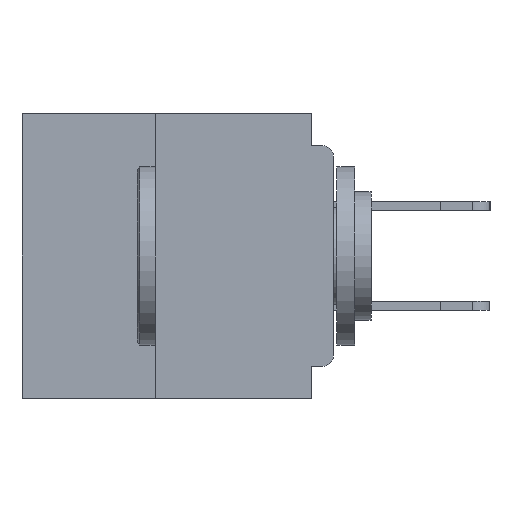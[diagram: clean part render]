
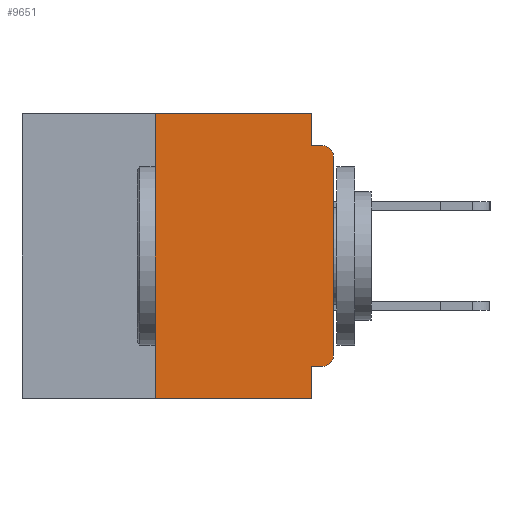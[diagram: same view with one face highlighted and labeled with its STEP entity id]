
A CAD part, left-side view. The second image highlights one B-rep face of the part: STEP entity #9651.
In plain terms, the highlighted planar face has unit normal (-1, 0, 0).
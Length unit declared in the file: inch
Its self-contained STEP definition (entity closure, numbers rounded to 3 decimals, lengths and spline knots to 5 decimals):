
#902 = VECTOR ( 'NONE', #10446, 39.37008 ) ;
#957 = EDGE_CURVE ( 'NONE', #3552, #12985, #12526, .T. ) ;
#1160 = DIRECTION ( 'NONE',  ( 0., 0., -1. ) ) ;
#1739 = EDGE_CURVE ( 'NONE', #25780, #27255, #29302, .T. ) ;
#3304 = CARTESIAN_POINT ( 'NONE',  ( 0., 0.437, 0. ) ) ;
#3520 = CIRCLE ( 'NONE', #38357, 0.015 ) ;
#3552 = VERTEX_POINT ( 'NONE', #10117 ) ;
#4319 = ORIENTED_EDGE ( 'NONE', *, *, #46952, .T. ) ;
#4646 = CIRCLE ( 'NONE', #32870, 0.015 ) ;
#4761 = CARTESIAN_POINT ( 'NONE',  ( 0., 0.437, 0. ) ) ;
#5683 = DIRECTION ( 'NONE',  ( 0., 0., 1. ) ) ;
#7208 = VECTOR ( 'NONE', #29849, 39.37008 ) ;
#7332 = DIRECTION ( 'NONE',  ( 0., 0., -1. ) ) ;
#8312 = ORIENTED_EDGE ( 'NONE', *, *, #50219, .T. ) ;
#9651 = ADVANCED_FACE ( 'NONE', ( #43883 ), #39194, .F. ) ;
#10117 = CARTESIAN_POINT ( 'NONE',  ( 0., 0.015, -0.355 ) ) ;
#10415 = VECTOR ( 'NONE', #1160, 39.37008 ) ;
#10446 = DIRECTION ( 'NONE',  ( 0., 0., 1. ) ) ;
#11949 = CARTESIAN_POINT ( 'NONE',  ( 0., 0.031, 0. ) ) ;
#12032 = CARTESIAN_POINT ( 'NONE',  ( 0., 0.031, 0. ) ) ;
#12138 = DIRECTION ( 'NONE',  ( 0., 0., -1. ) ) ;
#12167 = CARTESIAN_POINT ( 'NONE',  ( 0., 0.031, -0.045 ) ) ;
#12526 = LINE ( 'NONE', #34211, #32506 ) ;
#12985 = VERTEX_POINT ( 'NONE', #25009 ) ;
#13165 = CARTESIAN_POINT ( 'NONE',  ( 0., 0.015, -0.34 ) ) ;
#13362 = CARTESIAN_POINT ( 'NONE',  ( 0., 0.25, 0. ) ) ;
#13666 = CARTESIAN_POINT ( 'NONE',  ( 0., 0., -0.34 ) ) ;
#16185 = ORIENTED_EDGE ( 'NONE', *, *, #16230, .F. ) ;
#16230 = EDGE_CURVE ( 'NONE', #12985, #46934, #42355, .T. ) ;
#17060 = ORIENTED_EDGE ( 'NONE', *, *, #30318, .T. ) ;
#17192 = CARTESIAN_POINT ( 'NONE',  ( 0., 0.031, -0.4 ) ) ;
#17198 = DIRECTION ( 'NONE',  ( 0., 0., -1. ) ) ;
#18557 = LINE ( 'NONE', #4761, #30383 ) ;
#21283 = VERTEX_POINT ( 'NONE', #22860 ) ;
#22087 = DIRECTION ( 'NONE',  ( -1., 0., 0. ) ) ;
#22860 = CARTESIAN_POINT ( 'NONE',  ( 0., 0., -0.06 ) ) ;
#23069 = EDGE_CURVE ( 'NONE', #38877, #38316, #24604, .T. ) ;
#23240 = ORIENTED_EDGE ( 'NONE', *, *, #49475, .F. ) ;
#24604 = LINE ( 'NONE', #49763, #42113 ) ;
#25009 = CARTESIAN_POINT ( 'NONE',  ( 0., 0.031, -0.355 ) ) ;
#25780 = VERTEX_POINT ( 'NONE', #11949 ) ;
#26071 = VERTEX_POINT ( 'NONE', #31983 ) ;
#27215 = ORIENTED_EDGE ( 'NONE', *, *, #957, .F. ) ;
#27255 = VERTEX_POINT ( 'NONE', #12167 ) ;
#28062 = VECTOR ( 'NONE', #12138, 39.37008 ) ;
#28216 = ORIENTED_EDGE ( 'NONE', *, *, #1739, .F. ) ;
#29186 = LINE ( 'NONE', #42263, #50502 ) ;
#29302 = LINE ( 'NONE', #12032, #28062 ) ;
#29849 = DIRECTION ( 'NONE',  ( 0., -1., 0. ) ) ;
#30170 = CARTESIAN_POINT ( 'NONE',  ( 0., 0.031, -0.4 ) ) ;
#30318 = EDGE_CURVE ( 'NONE', #31429, #21283, #30384, .T. ) ;
#30383 = VECTOR ( 'NONE', #32729, 39.37008 ) ;
#30384 = LINE ( 'NONE', #34423, #902 ) ;
#30903 = AXIS2_PLACEMENT_3D ( 'NONE', #3304, #31277, #7332 ) ;
#31277 = DIRECTION ( 'NONE',  ( 1., 0., 0. ) ) ;
#31347 = EDGE_CURVE ( 'NONE', #3552, #31429, #3520, .T. ) ;
#31429 = VERTEX_POINT ( 'NONE', #13666 ) ;
#31983 = CARTESIAN_POINT ( 'NONE',  ( 0., 0.015, -0.045 ) ) ;
#32133 = EDGE_CURVE ( 'NONE', #27255, #26071, #39153, .T. ) ;
#32506 = VECTOR ( 'NONE', #33987, 39.37008 ) ;
#32729 = DIRECTION ( 'NONE',  ( 0., -1., 0. ) ) ;
#32870 = AXIS2_PLACEMENT_3D ( 'NONE', #46034, #22087, #50019 ) ;
#33987 = DIRECTION ( 'NONE',  ( 0., 1., 0. ) ) ;
#34211 = CARTESIAN_POINT ( 'NONE',  ( 0., 0., -0.355 ) ) ;
#34423 = CARTESIAN_POINT ( 'NONE',  ( 0., 0., 0. ) ) ;
#35815 = ORIENTED_EDGE ( 'NONE', *, *, #31347, .T. ) ;
#38316 = VERTEX_POINT ( 'NONE', #13362 ) ;
#38357 = AXIS2_PLACEMENT_3D ( 'NONE', #13165, #41129, #17198 ) ;
#38877 = VERTEX_POINT ( 'NONE', #45164 ) ;
#39153 = LINE ( 'NONE', #49815, #7208 ) ;
#39194 = PLANE ( 'NONE',  #30903 ) ;
#41129 = DIRECTION ( 'NONE',  ( -1., 0., 0. ) ) ;
#42113 = VECTOR ( 'NONE', #5683, 39.37008 ) ;
#42263 = CARTESIAN_POINT ( 'NONE',  ( 0., 0.437, -0.4 ) ) ;
#42355 = LINE ( 'NONE', #17192, #10415 ) ;
#42460 = ORIENTED_EDGE ( 'NONE', *, *, #23069, .F. ) ;
#43883 = FACE_OUTER_BOUND ( 'NONE', #51562, .T. ) ;
#45164 = CARTESIAN_POINT ( 'NONE',  ( 0., 0.25, -0.4 ) ) ;
#46034 = CARTESIAN_POINT ( 'NONE',  ( 0., 0.015, -0.06 ) ) ;
#46317 = DIRECTION ( 'NONE',  ( 0., -1., 0. ) ) ;
#46934 = VERTEX_POINT ( 'NONE', #30170 ) ;
#46952 = EDGE_CURVE ( 'NONE', #38877, #46934, #29186, .T. ) ;
#49475 = EDGE_CURVE ( 'NONE', #38316, #25780, #18557, .T. ) ;
#49763 = CARTESIAN_POINT ( 'NONE',  ( 0., 0.25, -0.4 ) ) ;
#49815 = CARTESIAN_POINT ( 'NONE',  ( 0., 0., -0.045 ) ) ;
#50019 = DIRECTION ( 'NONE',  ( 0., 0., -1. ) ) ;
#50219 = EDGE_CURVE ( 'NONE', #21283, #26071, #4646, .T. ) ;
#50502 = VECTOR ( 'NONE', #46317, 39.37008 ) ;
#51007 = ORIENTED_EDGE ( 'NONE', *, *, #32133, .F. ) ;
#51562 = EDGE_LOOP ( 'NONE', ( #17060, #8312, #51007, #28216, #23240, #42460, #4319, #16185, #27215, #35815 ) ) ;
